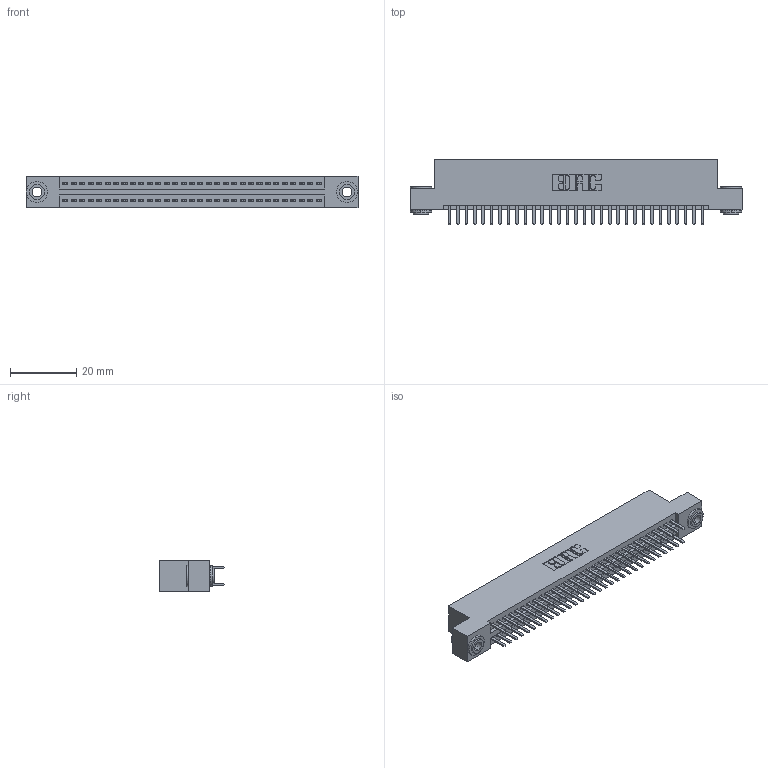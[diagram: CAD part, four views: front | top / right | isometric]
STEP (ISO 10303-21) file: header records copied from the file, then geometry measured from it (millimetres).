
FILE_DESCRIPTION (( 'STEP AP203' ), '1' );
FILE_NAME ('395-062-520-203.STEP', '2018-11-23T23:50:27', ( '' ), ( '' ), 'SwSTEP 2.0', 'SolidWorks 2016', '' );
FILE_SCHEMA (( 'CONFIG_CONTROL_DESIGN' ));
Length unit declared in the file: inch
Products named in the file (4): 345-250-002_345-250-002-102; 395-062-520-203; 345 Part_Flush Mounting Lugs - 0.156 Dia-TH; 345-292-001_345-293-120
Assembly tree (65 placements, depth 2):
  395-062-520-203
    345 Part_Flush Mounting Lugs - 0.156 Dia-TH
    345-292-001_345-293-120  x62
    345-250-002_345-250-002-102  x2
Bounding box: 99.95 x 19.68 x 9.4 mm (x, y, z)
Volume: 9599.2 mm3; surface area: 14123.1 mm2
Topology: 65 solids, 65 shells, 3512 faces, 10151 edges, 6598 vertices
Faces by surface type: plane 2260, cylinder 1244, cone 8
Entity records: 26568 total; most frequent: CARTESIAN_POINT 4451, ORIENTED_EDGE 4366, DIRECTION 3957, EDGE_CURVE 2183, LINE 1899, VECTOR 1899, VERTEX_POINT 1450, AXIS2_PLACEMENT_3D 1029
